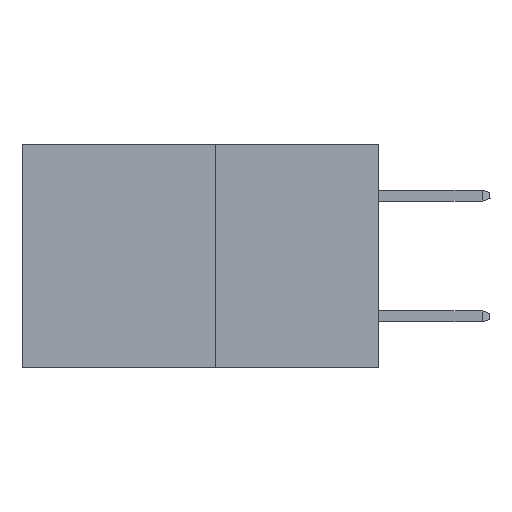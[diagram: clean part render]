
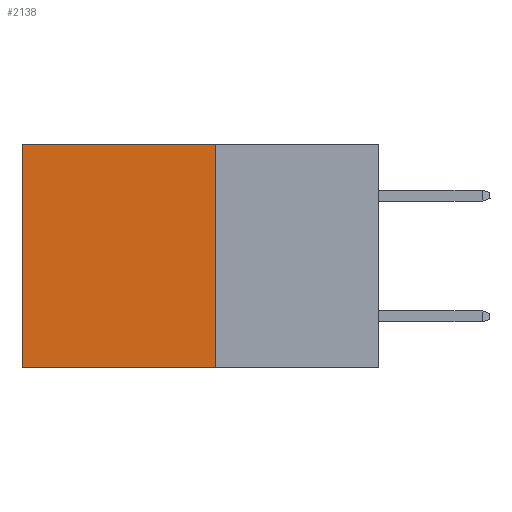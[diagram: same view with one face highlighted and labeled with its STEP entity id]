
A CAD part, left-side view. The second image highlights one B-rep face of the part: STEP entity #2138.
In plain terms, the highlighted planar face has unit normal (-1, 0, 0).
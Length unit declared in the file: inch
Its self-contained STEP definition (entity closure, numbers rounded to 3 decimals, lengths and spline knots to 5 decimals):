
#514 = ORIENTED_EDGE ( 'NONE', *, *, #5785, .T. ) ;
#526 = LINE ( 'NONE', #983, #5913 ) ;
#678 = DIRECTION ( 'NONE',  ( 0., 0., -1. ) ) ;
#694 = ORIENTED_EDGE ( 'NONE', *, *, #2109, .F. ) ;
#727 = ORIENTED_EDGE ( 'NONE', *, *, #5330, .F. ) ;
#863 = ORIENTED_EDGE ( 'NONE', *, *, #3605, .T. ) ;
#983 = CARTESIAN_POINT ( 'NONE',  ( 0.277, 0.59, -0.37 ) ) ;
#1015 = VERTEX_POINT ( 'NONE', #1079 ) ;
#1079 = CARTESIAN_POINT ( 'NONE',  ( 0.277, 0.59, -0.37 ) ) ;
#1951 = VECTOR ( 'NONE', #2313, 39.37008 ) ;
#2014 = DIRECTION ( 'NONE',  ( 0., 1., 0. ) ) ;
#2109 = EDGE_CURVE ( 'NONE', #2749, #1015, #4972, .T. ) ;
#2138 = ADVANCED_FACE ( 'NONE', ( #6407 ), #4323, .F. ) ;
#2313 = DIRECTION ( 'NONE',  ( 0., 0., -1. ) ) ;
#2541 = VERTEX_POINT ( 'NONE', #8112 ) ;
#2671 = EDGE_LOOP ( 'NONE', ( #514, #694, #727, #863 ) ) ;
#2749 = VERTEX_POINT ( 'NONE', #6687 ) ;
#3605 = EDGE_CURVE ( 'NONE', #2541, #5949, #8599, .T. ) ;
#4025 = LINE ( 'NONE', #5342, #1951 ) ;
#4323 = PLANE ( 'NONE',  #7072 ) ;
#4972 = LINE ( 'NONE', #6461, #8315 ) ;
#5330 = EDGE_CURVE ( 'NONE', #2541, #2749, #4025, .T. ) ;
#5342 = CARTESIAN_POINT ( 'NONE',  ( 0.277, 0.27, -0.37 ) ) ;
#5785 = EDGE_CURVE ( 'NONE', #5949, #1015, #526, .T. ) ;
#5905 = DIRECTION ( 'NONE',  ( 0., 0., -1. ) ) ;
#5913 = VECTOR ( 'NONE', #678, 39.37008 ) ;
#5949 = VERTEX_POINT ( 'NONE', #8735 ) ;
#6191 = DIRECTION ( 'NONE',  ( 1., 0., 0. ) ) ;
#6407 = FACE_OUTER_BOUND ( 'NONE', #2671, .T. ) ;
#6461 = CARTESIAN_POINT ( 'NONE',  ( 0.277, 0.27, -0.37 ) ) ;
#6687 = CARTESIAN_POINT ( 'NONE',  ( 0.277, 0.27, -0.37 ) ) ;
#7072 = AXIS2_PLACEMENT_3D ( 'NONE', #8713, #6191, #5905 ) ;
#7867 = CARTESIAN_POINT ( 'NONE',  ( 0.277, 0.27, 0. ) ) ;
#7874 = DIRECTION ( 'NONE',  ( 0., 1., 0. ) ) ;
#8112 = CARTESIAN_POINT ( 'NONE',  ( 0.277, 0.27, 0. ) ) ;
#8210 = VECTOR ( 'NONE', #7874, 39.37008 ) ;
#8315 = VECTOR ( 'NONE', #2014, 39.37008 ) ;
#8599 = LINE ( 'NONE', #7867, #8210 ) ;
#8713 = CARTESIAN_POINT ( 'NONE',  ( 0.277, 0.27, -0.37 ) ) ;
#8735 = CARTESIAN_POINT ( 'NONE',  ( 0.277, 0.59, 0. ) ) ;
